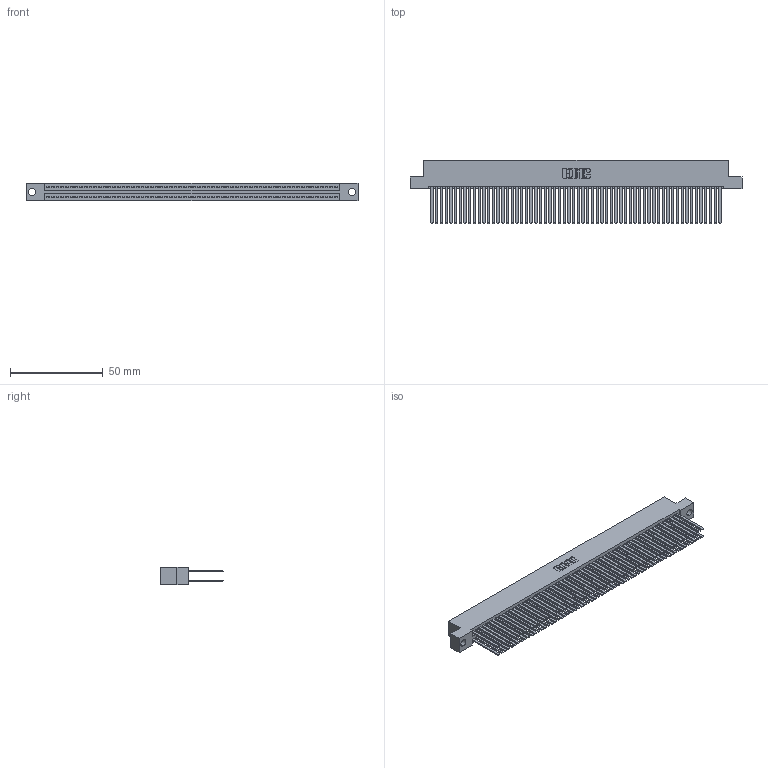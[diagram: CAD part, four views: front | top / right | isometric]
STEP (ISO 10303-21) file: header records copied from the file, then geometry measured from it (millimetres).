
FILE_DESCRIPTION (( 'STEP AP203' ), '1' );
FILE_NAME ('395-124-544-204.STEP', '2021-06-17T22:15:38', ( '' ), ( '' ), 'SwSTEP 2.0', 'SolidWorks 2020', '' );
FILE_SCHEMA (( 'CONFIG_CONTROL_DESIGN' ));
Length unit declared in the file: inch
Products named in the file (3): 345-292-001_345-293-144; 345 Part_Flush Mounting Lugs - 0.156 Dia-TI; 395-124-544-204
Assembly tree (125 placements, depth 2):
  395-124-544-204
    345 Part_Flush Mounting Lugs - 0.156 Dia-TI
    345-292-001_345-293-144  x124
Bounding box: 178.69 x 33.96 x 9.4 mm (x, y, z)
Volume: 19176 mm3; surface area: 33678.9 mm2
Topology: 125 solids, 125 shells, 5596 faces, 16621 edges, 10914 vertices
Faces by surface type: plane 3690, cylinder 1906
Entity records: 46189 total; most frequent: CARTESIAN_POINT 7726, ORIENTED_EDGE 7658, DIRECTION 6785, EDGE_CURVE 3829, VECTOR 3453, LINE 3453, VERTEX_POINT 2550, AXIS2_PLACEMENT_3D 1666
